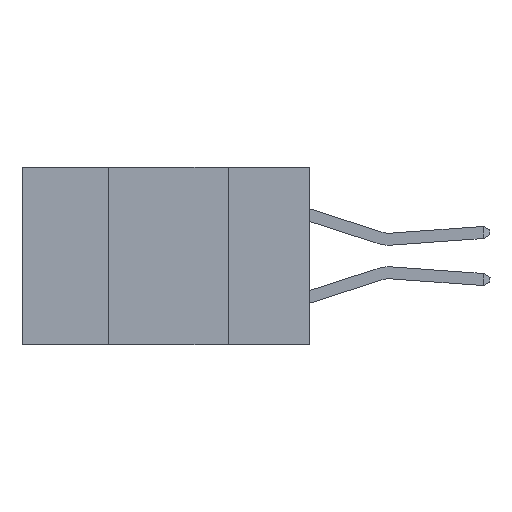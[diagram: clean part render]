
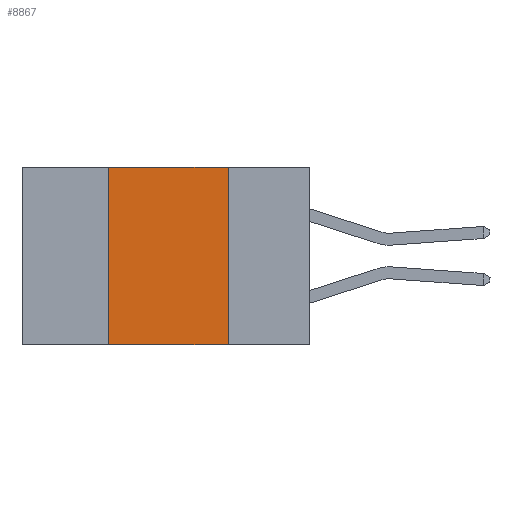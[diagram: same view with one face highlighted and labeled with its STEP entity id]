
A CAD part, left-side view. The second image highlights one B-rep face of the part: STEP entity #8867.
In plain terms, the highlighted planar face has unit normal (-1, 0, 0).
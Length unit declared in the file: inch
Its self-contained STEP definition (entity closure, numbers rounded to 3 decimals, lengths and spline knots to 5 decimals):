
#21 = CARTESIAN_POINT ( 'NONE',  ( 0., 0.17, -0.37 ) ) ;
#143 = CARTESIAN_POINT ( 'NONE',  ( 0., 0.6, 0. ) ) ;
#417 = ORIENTED_EDGE ( 'NONE', *, *, #946, .F. ) ;
#655 = EDGE_LOOP ( 'NONE', ( #13533, #13929, #417, #4291 ) ) ;
#700 = DIRECTION ( 'NONE',  ( 0., 0., -1. ) ) ;
#946 = EDGE_CURVE ( 'NONE', #9672, #11578, #3646, .T. ) ;
#1087 = VERTEX_POINT ( 'NONE', #2246 ) ;
#1358 = AXIS2_PLACEMENT_3D ( 'NONE', #9839, #6635, #4484 ) ;
#2246 = CARTESIAN_POINT ( 'NONE',  ( 0., 0.17, 0. ) ) ;
#2347 = PLANE ( 'NONE',  #1358 ) ;
#2416 = DIRECTION ( 'NONE',  ( 0., 0., 1. ) ) ;
#2478 = LINE ( 'NONE', #4753, #9360 ) ;
#2909 = CARTESIAN_POINT ( 'NONE',  ( 0., 0.17, 0. ) ) ;
#3398 = VECTOR ( 'NONE', #700, 39.37008 ) ;
#3646 = LINE ( 'NONE', #4685, #10543 ) ;
#4291 = ORIENTED_EDGE ( 'NONE', *, *, #7496, .T. ) ;
#4301 = VERTEX_POINT ( 'NONE', #21 ) ;
#4484 = DIRECTION ( 'NONE',  ( 0., 0., -1. ) ) ;
#4685 = CARTESIAN_POINT ( 'NONE',  ( 0., 0.42, 0. ) ) ;
#4753 = CARTESIAN_POINT ( 'NONE',  ( 0., 0.6, -0.37 ) ) ;
#5137 = VECTOR ( 'NONE', #5598, 39.37008 ) ;
#5598 = DIRECTION ( 'NONE',  ( 0., -1., 0. ) ) ;
#6635 = DIRECTION ( 'NONE',  ( 1., 0., 0. ) ) ;
#7282 = LINE ( 'NONE', #2909, #3398 ) ;
#7496 = EDGE_CURVE ( 'NONE', #9672, #4301, #2478, .T. ) ;
#7981 = FACE_OUTER_BOUND ( 'NONE', #655, .T. ) ;
#8142 = LINE ( 'NONE', #143, #5137 ) ;
#8867 = ADVANCED_FACE ( 'NONE', ( #7981 ), #2347, .F. ) ;
#9069 = CARTESIAN_POINT ( 'NONE',  ( 0., 0.42, -0.37 ) ) ;
#9360 = VECTOR ( 'NONE', #12330, 39.37008 ) ;
#9672 = VERTEX_POINT ( 'NONE', #9069 ) ;
#9839 = CARTESIAN_POINT ( 'NONE',  ( 0., 0.6, 0. ) ) ;
#10543 = VECTOR ( 'NONE', #2416, 39.37008 ) ;
#11578 = VERTEX_POINT ( 'NONE', #12187 ) ;
#12105 = EDGE_CURVE ( 'NONE', #11578, #1087, #8142, .T. ) ;
#12187 = CARTESIAN_POINT ( 'NONE',  ( 0., 0.42, 0. ) ) ;
#12330 = DIRECTION ( 'NONE',  ( 0., -1., 0. ) ) ;
#13533 = ORIENTED_EDGE ( 'NONE', *, *, #13960, .F. ) ;
#13929 = ORIENTED_EDGE ( 'NONE', *, *, #12105, .F. ) ;
#13960 = EDGE_CURVE ( 'NONE', #1087, #4301, #7282, .T. ) ;
